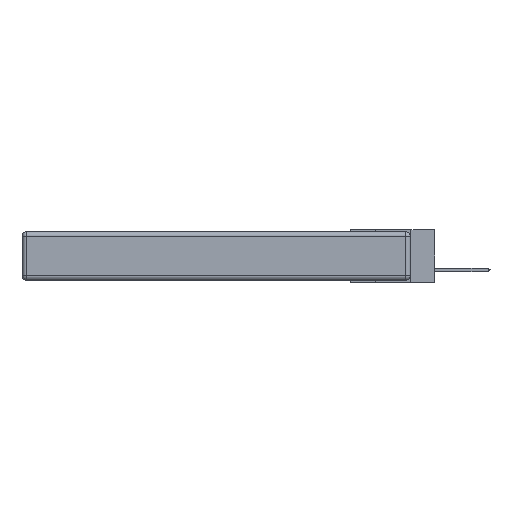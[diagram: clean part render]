
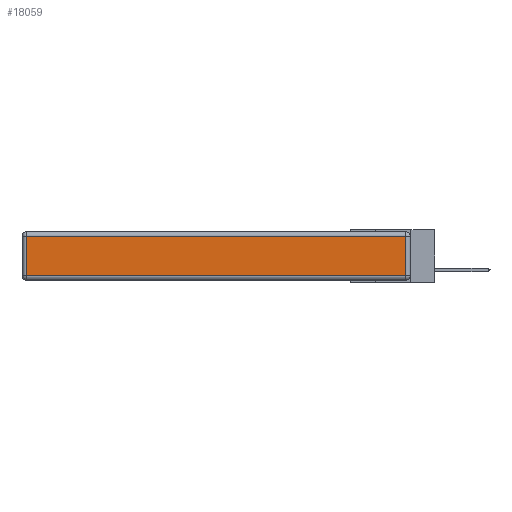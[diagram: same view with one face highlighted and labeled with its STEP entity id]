
A CAD part, left-side view. The second image highlights one B-rep face of the part: STEP entity #18059.
In plain terms, the highlighted planar face has unit normal (-1, 0, 0).
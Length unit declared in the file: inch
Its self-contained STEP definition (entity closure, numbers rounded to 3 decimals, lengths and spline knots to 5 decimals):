
#380 = CARTESIAN_POINT ( 'NONE',  ( 0., 2.72, -0.313 ) ) ;
#499 = LINE ( 'NONE', #21939, #16810 ) ;
#585 = VECTOR ( 'NONE', #14848, 39.37008 ) ;
#1090 = DIRECTION ( 'NONE',  ( 0., 0., -1. ) ) ;
#1423 = DIRECTION ( 'NONE',  ( 0., -1., 0. ) ) ;
#1439 = LINE ( 'NONE', #9455, #585 ) ;
#1735 = LINE ( 'NONE', #18070, #10911 ) ;
#1758 = CARTESIAN_POINT ( 'NONE',  ( 0., 0., -0.313 ) ) ;
#3045 = ORIENTED_EDGE ( 'NONE', *, *, #6658, .T. ) ;
#3656 = CARTESIAN_POINT ( 'NONE',  ( 0., 0.03, -0.03 ) ) ;
#4254 = EDGE_CURVE ( 'NONE', #5150, #27105, #1735, .T. ) ;
#5150 = VERTEX_POINT ( 'NONE', #17883 ) ;
#6166 = EDGE_LOOP ( 'NONE', ( #16145, #29661, #16621, #3045 ) ) ;
#6658 = EDGE_CURVE ( 'NONE', #7321, #7650, #499, .T. ) ;
#7321 = VERTEX_POINT ( 'NONE', #10440 ) ;
#7650 = VERTEX_POINT ( 'NONE', #380 ) ;
#7922 = CARTESIAN_POINT ( 'NONE',  ( 0., 0., -0.343 ) ) ;
#8030 = DIRECTION ( 'NONE',  ( -1., 0., 0. ) ) ;
#9455 = CARTESIAN_POINT ( 'NONE',  ( 0., 2.75, -0.03 ) ) ;
#10440 = CARTESIAN_POINT ( 'NONE',  ( 0., 2.72, -0.03 ) ) ;
#10911 = VECTOR ( 'NONE', #21034, 39.37008 ) ;
#14848 = DIRECTION ( 'NONE',  ( 0., 1., 0. ) ) ;
#15651 = PLANE ( 'NONE',  #20906 ) ;
#16145 = ORIENTED_EDGE ( 'NONE', *, *, #20130, .T. ) ;
#16621 = ORIENTED_EDGE ( 'NONE', *, *, #28482, .T. ) ;
#16810 = VECTOR ( 'NONE', #1090, 39.37008 ) ;
#17883 = CARTESIAN_POINT ( 'NONE',  ( 0., 0.03, -0.313 ) ) ;
#18059 = ADVANCED_FACE ( 'NONE', ( #30025 ), #15651, .T. ) ;
#18070 = CARTESIAN_POINT ( 'NONE',  ( 0., 0.03, -0.343 ) ) ;
#19553 = VECTOR ( 'NONE', #1423, 39.37008 ) ;
#20130 = EDGE_CURVE ( 'NONE', #7650, #5150, #21245, .T. ) ;
#20906 = AXIS2_PLACEMENT_3D ( 'NONE', #7922, #8030, #23765 ) ;
#21034 = DIRECTION ( 'NONE',  ( 0., 0., 1. ) ) ;
#21245 = LINE ( 'NONE', #1758, #19553 ) ;
#21939 = CARTESIAN_POINT ( 'NONE',  ( 0., 2.72, -0.343 ) ) ;
#23765 = DIRECTION ( 'NONE',  ( 0., 0., 1. ) ) ;
#27105 = VERTEX_POINT ( 'NONE', #3656 ) ;
#28482 = EDGE_CURVE ( 'NONE', #27105, #7321, #1439, .T. ) ;
#29661 = ORIENTED_EDGE ( 'NONE', *, *, #4254, .T. ) ;
#30025 = FACE_OUTER_BOUND ( 'NONE', #6166, .T. ) ;
